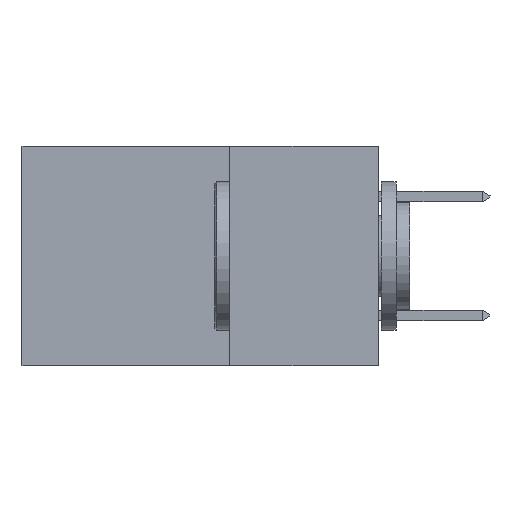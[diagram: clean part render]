
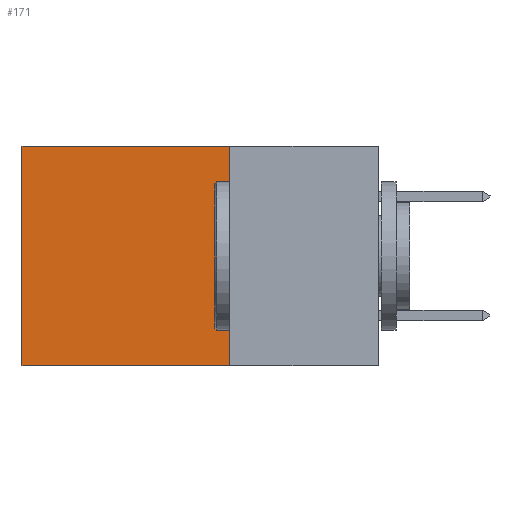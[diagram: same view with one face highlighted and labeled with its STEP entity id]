
A CAD part, left-side view. The second image highlights one B-rep face of the part: STEP entity #171.
In plain terms, the highlighted planar face has unit normal (-1, 0, 0).
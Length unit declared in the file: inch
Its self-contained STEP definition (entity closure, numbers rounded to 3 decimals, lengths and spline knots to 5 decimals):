
#171 = ADVANCED_FACE ( 'NONE', ( #1117 ), #6057, .F. ) ;
#245 = DIRECTION ( 'NONE',  ( 0., 0., -1. ) ) ;
#272 = ORIENTED_EDGE ( 'NONE', *, *, #2461, .F. ) ;
#305 = DIRECTION ( 'NONE',  ( 0., 1., 0. ) ) ;
#1117 = FACE_OUTER_BOUND ( 'NONE', #10402, .T. ) ;
#1178 = LINE ( 'NONE', #6058, #4132 ) ;
#1216 = VECTOR ( 'NONE', #8090, 39.37008 ) ;
#2115 = DIRECTION ( 'NONE',  ( 0., 1., 0. ) ) ;
#2231 = AXIS2_PLACEMENT_3D ( 'NONE', #7892, #10293, #245 ) ;
#2267 = LINE ( 'NONE', #7319, #3119 ) ;
#2461 = EDGE_CURVE ( 'NONE', #9156, #9460, #7049, .T. ) ;
#3119 = VECTOR ( 'NONE', #2115, 39.37008 ) ;
#3772 = CARTESIAN_POINT ( 'NONE',  ( 0.2615, 0.6, -0.37 ) ) ;
#3783 = CARTESIAN_POINT ( 'NONE',  ( 0.2615, 0.6, -0.37 ) ) ;
#3798 = CARTESIAN_POINT ( 'NONE',  ( 0.2615, 0.25, -0.37 ) ) ;
#4132 = VECTOR ( 'NONE', #305, 39.37008 ) ;
#5372 = CARTESIAN_POINT ( 'NONE',  ( 0.2615, 0.6, 0. ) ) ;
#6057 = PLANE ( 'NONE',  #2231 ) ;
#6058 = CARTESIAN_POINT ( 'NONE',  ( 0.2615, 0.25, -0.37 ) ) ;
#6193 = LINE ( 'NONE', #3783, #6430 ) ;
#6430 = VECTOR ( 'NONE', #9547, 39.37008 ) ;
#7049 = LINE ( 'NONE', #3798, #1216 ) ;
#7319 = CARTESIAN_POINT ( 'NONE',  ( 0.2615, 0.25, 0. ) ) ;
#7363 = VERTEX_POINT ( 'NONE', #5372 ) ;
#7641 = EDGE_CURVE ( 'NONE', #9460, #9027, #1178, .T. ) ;
#7657 = ORIENTED_EDGE ( 'NONE', *, *, #8480, .T. ) ;
#7892 = CARTESIAN_POINT ( 'NONE',  ( 0.2615, 0.25, -0.37 ) ) ;
#8090 = DIRECTION ( 'NONE',  ( 0., 0., -1. ) ) ;
#8333 = ORIENTED_EDGE ( 'NONE', *, *, #7641, .F. ) ;
#8382 = CARTESIAN_POINT ( 'NONE',  ( 0.2615, 0.25, 0. ) ) ;
#8480 = EDGE_CURVE ( 'NONE', #7363, #9027, #6193, .T. ) ;
#8664 = ORIENTED_EDGE ( 'NONE', *, *, #9852, .T. ) ;
#9027 = VERTEX_POINT ( 'NONE', #3772 ) ;
#9156 = VERTEX_POINT ( 'NONE', #8382 ) ;
#9460 = VERTEX_POINT ( 'NONE', #10625 ) ;
#9547 = DIRECTION ( 'NONE',  ( 0., 0., -1. ) ) ;
#9852 = EDGE_CURVE ( 'NONE', #9156, #7363, #2267, .T. ) ;
#10293 = DIRECTION ( 'NONE',  ( 1., 0., 0. ) ) ;
#10402 = EDGE_LOOP ( 'NONE', ( #7657, #8333, #272, #8664 ) ) ;
#10625 = CARTESIAN_POINT ( 'NONE',  ( 0.2615, 0.25, -0.37 ) ) ;
